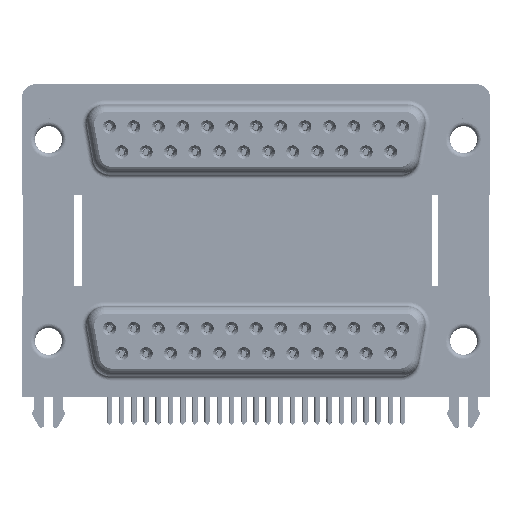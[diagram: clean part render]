
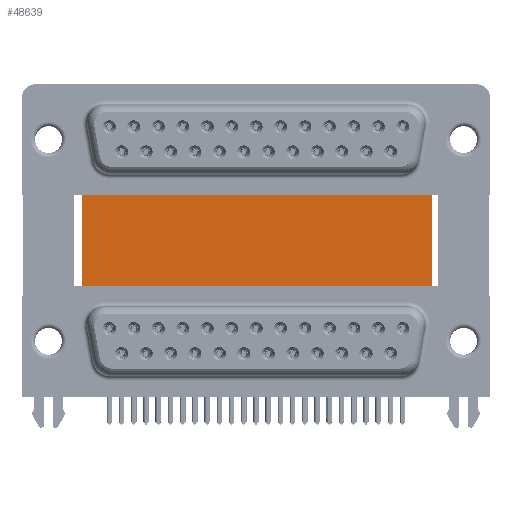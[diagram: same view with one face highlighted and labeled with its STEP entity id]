
A CAD part, top view. The second image highlights one B-rep face of the part: STEP entity #48639.
In plain terms, the highlighted planar face has unit normal (0, 0, 1).
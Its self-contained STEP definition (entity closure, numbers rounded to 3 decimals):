
#163 = LINE ( 'NONE', #41587, #26825 ) ;
#408 = VERTEX_POINT ( 'NONE', #8250 ) ;
#1084 = DIRECTION ( 'NONE',  ( -1., 0., 0. ) ) ;
#6852 = DIRECTION ( 'NONE',  ( 1., 0., 0. ) ) ;
#7387 = LINE ( 'NONE', #11403, #60227 ) ;
#7420 = ORIENTED_EDGE ( 'NONE', *, *, #26358, .T. ) ;
#8250 = CARTESIAN_POINT ( 'NONE',  ( 3.79, -3.735, -12. ) ) ;
#8333 = EDGE_LOOP ( 'NONE', ( #7420, #27226, #27031, #13400 ) ) ;
#9744 = CARTESIAN_POINT ( 'NONE',  ( 43.43, 16.585, -12. ) ) ;
#10300 = DIRECTION ( 'NONE',  ( 1., 0., 0. ) ) ;
#11403 = CARTESIAN_POINT ( 'NONE',  ( 43.43, 16.585, -12. ) ) ;
#13270 = VERTEX_POINT ( 'NONE', #30562 ) ;
#13400 = ORIENTED_EDGE ( 'NONE', *, *, #21447, .T. ) ;
#15836 = LINE ( 'NONE', #56966, #32236 ) ;
#17982 = DIRECTION ( 'NONE',  ( 0., -1., 0. ) ) ;
#20138 = DIRECTION ( 'NONE',  ( 0., 0., -1. ) ) ;
#21447 = EDGE_CURVE ( 'NONE', #13270, #408, #163, .T. ) ;
#23283 = EDGE_CURVE ( 'NONE', #49419, #38826, #7387, .T. ) ;
#25355 = PLANE ( 'NONE',  #33680 ) ;
#26358 = EDGE_CURVE ( 'NONE', #408, #38826, #48920, .T. ) ;
#26825 = VECTOR ( 'NONE', #17982, 1000. ) ;
#27031 = ORIENTED_EDGE ( 'NONE', *, *, #28770, .F. ) ;
#27226 = ORIENTED_EDGE ( 'NONE', *, *, #23283, .F. ) ;
#28770 = EDGE_CURVE ( 'NONE', #13270, #49419, #15836, .T. ) ;
#30203 = CARTESIAN_POINT ( 'NONE',  ( 3.79, -3.735, -12. ) ) ;
#30562 = CARTESIAN_POINT ( 'NONE',  ( 3.79, 16.585, -12. ) ) ;
#32236 = VECTOR ( 'NONE', #10300, 1000. ) ;
#33680 = AXIS2_PLACEMENT_3D ( 'NONE', #46587, #20138, #1084 ) ;
#35614 = CARTESIAN_POINT ( 'NONE',  ( 43.43, -3.735, -12. ) ) ;
#35623 = DIRECTION ( 'NONE',  ( 0., -1., 0. ) ) ;
#38826 = VERTEX_POINT ( 'NONE', #35614 ) ;
#41587 = CARTESIAN_POINT ( 'NONE',  ( 3.79, 16.585, -12. ) ) ;
#43121 = FACE_OUTER_BOUND ( 'NONE', #8333, .T. ) ;
#46587 = CARTESIAN_POINT ( 'NONE',  ( 3.79, 16.585, -12. ) ) ;
#48639 = ADVANCED_FACE ( 'NONE', ( #43121 ), #25355, .F. ) ;
#48920 = LINE ( 'NONE', #30203, #57412 ) ;
#49419 = VERTEX_POINT ( 'NONE', #9744 ) ;
#56966 = CARTESIAN_POINT ( 'NONE',  ( 3.79, 16.585, -12. ) ) ;
#57412 = VECTOR ( 'NONE', #6852, 1000. ) ;
#60227 = VECTOR ( 'NONE', #35623, 1000. ) ;
